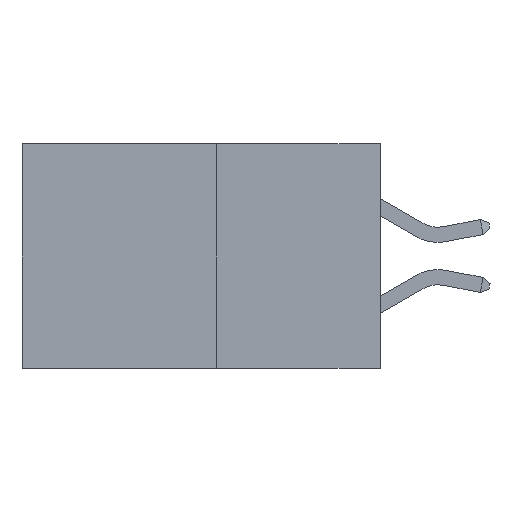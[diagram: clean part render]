
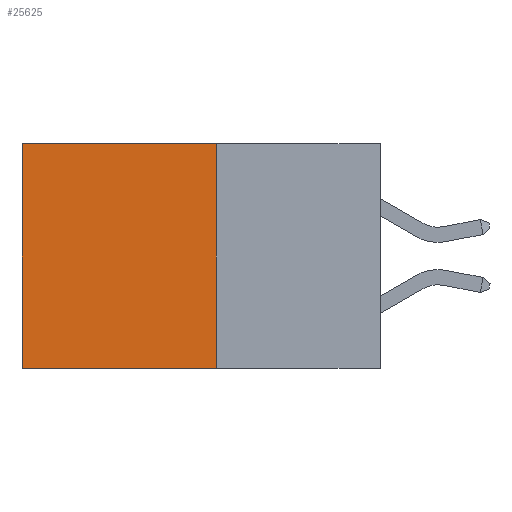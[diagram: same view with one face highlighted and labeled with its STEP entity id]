
A CAD part, left-side view. The second image highlights one B-rep face of the part: STEP entity #25625.
In plain terms, the highlighted planar face has unit normal (-1, 0, 0).
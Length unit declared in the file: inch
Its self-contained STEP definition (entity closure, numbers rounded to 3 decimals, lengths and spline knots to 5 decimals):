
#1530 = VERTEX_POINT ( 'NONE', #21524 ) ;
#1636 = EDGE_CURVE ( 'NONE', #1530, #25741, #25365, .T. ) ;
#1767 = AXIS2_PLACEMENT_3D ( 'NONE', #20721, #5024, #23324 ) ;
#1841 = VERTEX_POINT ( 'NONE', #14918 ) ;
#1927 = CARTESIAN_POINT ( 'NONE',  ( 0.277, 0.27, -0.37 ) ) ;
#3083 = EDGE_CURVE ( 'NONE', #1530, #23105, #18349, .T. ) ;
#5024 = DIRECTION ( 'NONE',  ( 1., 0., 0. ) ) ;
#5359 = VECTOR ( 'NONE', #21870, 39.37008 ) ;
#6042 = CARTESIAN_POINT ( 'NONE',  ( 0.277, 0.59, 0. ) ) ;
#7325 = DIRECTION ( 'NONE',  ( 0., 1., 0. ) ) ;
#7341 = VECTOR ( 'NONE', #12064, 39.37008 ) ;
#8555 = EDGE_LOOP ( 'NONE', ( #13372, #16888, #29866, #12756 ) ) ;
#10446 = VECTOR ( 'NONE', #7325, 39.37008 ) ;
#11280 = LINE ( 'NONE', #1927, #10446 ) ;
#12064 = DIRECTION ( 'NONE',  ( 0., 0., -1. ) ) ;
#12109 = CARTESIAN_POINT ( 'NONE',  ( 0.277, 0.59, -0.37 ) ) ;
#12756 = ORIENTED_EDGE ( 'NONE', *, *, #3083, .T. ) ;
#12893 = EDGE_CURVE ( 'NONE', #23105, #1841, #13478, .T. ) ;
#13372 = ORIENTED_EDGE ( 'NONE', *, *, #12893, .T. ) ;
#13478 = LINE ( 'NONE', #12109, #7341 ) ;
#14918 = CARTESIAN_POINT ( 'NONE',  ( 0.277, 0.59, -0.37 ) ) ;
#16888 = ORIENTED_EDGE ( 'NONE', *, *, #28038, .F. ) ;
#16939 = CARTESIAN_POINT ( 'NONE',  ( 0.277, 0.27, 0. ) ) ;
#17523 = VECTOR ( 'NONE', #28827, 39.37008 ) ;
#17742 = CARTESIAN_POINT ( 'NONE',  ( 0.277, 0.27, -0.37 ) ) ;
#18349 = LINE ( 'NONE', #16939, #17523 ) ;
#20721 = CARTESIAN_POINT ( 'NONE',  ( 0.277, 0.27, -0.37 ) ) ;
#21524 = CARTESIAN_POINT ( 'NONE',  ( 0.277, 0.27, 0. ) ) ;
#21870 = DIRECTION ( 'NONE',  ( 0., 0., -1. ) ) ;
#23105 = VERTEX_POINT ( 'NONE', #6042 ) ;
#23324 = DIRECTION ( 'NONE',  ( 0., 0., -1. ) ) ;
#24020 = FACE_OUTER_BOUND ( 'NONE', #8555, .T. ) ;
#25365 = LINE ( 'NONE', #17742, #5359 ) ;
#25625 = ADVANCED_FACE ( 'NONE', ( #24020 ), #30982, .F. ) ;
#25741 = VERTEX_POINT ( 'NONE', #26834 ) ;
#26834 = CARTESIAN_POINT ( 'NONE',  ( 0.277, 0.27, -0.37 ) ) ;
#28038 = EDGE_CURVE ( 'NONE', #25741, #1841, #11280, .T. ) ;
#28827 = DIRECTION ( 'NONE',  ( 0., 1., 0. ) ) ;
#29866 = ORIENTED_EDGE ( 'NONE', *, *, #1636, .F. ) ;
#30982 = PLANE ( 'NONE',  #1767 ) ;
